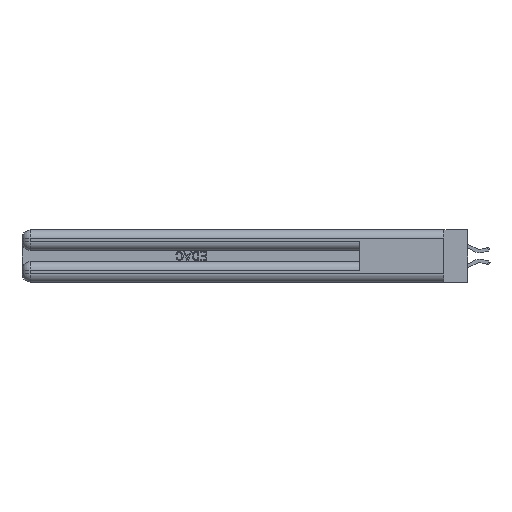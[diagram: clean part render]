
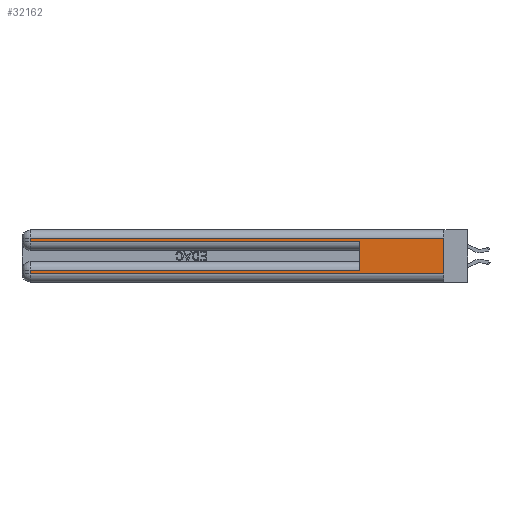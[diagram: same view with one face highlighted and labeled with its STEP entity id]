
A CAD part, left-side view. The second image highlights one B-rep face of the part: STEP entity #32162.
In plain terms, the highlighted planar face has unit normal (-1, 0, 0).
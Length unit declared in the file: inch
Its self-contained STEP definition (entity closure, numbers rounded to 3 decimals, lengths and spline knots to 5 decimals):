
#1844 = DIRECTION ( 'NONE',  ( 0., 0., -1. ) ) ;
#3125 = ORIENTED_EDGE ( 'NONE', *, *, #8062, .T. ) ;
#3623 = ORIENTED_EDGE ( 'NONE', *, *, #20312, .T. ) ;
#4975 = DIRECTION ( 'NONE',  ( 0., 0., -1. ) ) ;
#5886 = AXIS2_PLACEMENT_3D ( 'NONE', #33675, #36899, #17647 ) ;
#6478 = LINE ( 'NONE', #30797, #31210 ) ;
#6628 = LINE ( 'NONE', #17443, #39851 ) ;
#6711 = EDGE_CURVE ( 'NONE', #34396, #38334, #29450, .T. ) ;
#7261 = EDGE_CURVE ( 'NONE', #36686, #39911, #33912, .T. ) ;
#8062 = EDGE_CURVE ( 'NONE', #36686, #34396, #6628, .T. ) ;
#8280 = EDGE_LOOP ( 'NONE', ( #28367, #3623, #14246, #16308, #25900, #3125, #38433, #40405 ) ) ;
#9672 = VECTOR ( 'NONE', #1844, 39.37008 ) ;
#10663 = EDGE_CURVE ( 'NONE', #37939, #33189, #6478, .T. ) ;
#11004 = DIRECTION ( 'NONE',  ( 0., -1., 0. ) ) ;
#11037 = LINE ( 'NONE', #28527, #35695 ) ;
#11185 = PLANE ( 'NONE',  #5886 ) ;
#12347 = DIRECTION ( 'NONE',  ( 0., -1., 0. ) ) ;
#12499 = EDGE_CURVE ( 'NONE', #31010, #18338, #26779, .T. ) ;
#14246 = ORIENTED_EDGE ( 'NONE', *, *, #12499, .T. ) ;
#14874 = VECTOR ( 'NONE', #34053, 39.37008 ) ;
#16308 = ORIENTED_EDGE ( 'NONE', *, *, #22185, .T. ) ;
#17443 = CARTESIAN_POINT ( 'NONE',  ( 0., 0., 0.085 ) ) ;
#17647 = DIRECTION ( 'NONE',  ( 0., 0., -1. ) ) ;
#17827 = CARTESIAN_POINT ( 'NONE',  ( 0., 0.6, 0.145 ) ) ;
#17881 = CARTESIAN_POINT ( 'NONE',  ( 0., 0., 0.31 ) ) ;
#18338 = VERTEX_POINT ( 'NONE', #25374 ) ;
#19590 = CARTESIAN_POINT ( 'NONE',  ( 0., 2.94, 0.31 ) ) ;
#20312 = EDGE_CURVE ( 'NONE', #37939, #31010, #23450, .T. ) ;
#20659 = DIRECTION ( 'NONE',  ( 0., 1., 0. ) ) ;
#20880 = VECTOR ( 'NONE', #40449, 39.37008 ) ;
#22185 = EDGE_CURVE ( 'NONE', #18338, #39911, #30398, .T. ) ;
#22467 = FACE_OUTER_BOUND ( 'NONE', #8280, .T. ) ;
#22581 = CARTESIAN_POINT ( 'NONE',  ( 0., 2.94, 0.085 ) ) ;
#23450 = LINE ( 'NONE', #17881, #14874 ) ;
#23798 = CARTESIAN_POINT ( 'NONE',  ( 0., 0., 0.285 ) ) ;
#24309 = DIRECTION ( 'NONE',  ( 0., 0., 1. ) ) ;
#24623 = CARTESIAN_POINT ( 'NONE',  ( 0., 2.94, 0.37 ) ) ;
#25374 = CARTESIAN_POINT ( 'NONE',  ( 0., 2.94, 0.285 ) ) ;
#25411 = VECTOR ( 'NONE', #24309, 39.37008 ) ;
#25900 = ORIENTED_EDGE ( 'NONE', *, *, #7261, .F. ) ;
#26779 = LINE ( 'NONE', #24623, #9672 ) ;
#28060 = CARTESIAN_POINT ( 'NONE',  ( 0., 0.6, 0.285 ) ) ;
#28367 = ORIENTED_EDGE ( 'NONE', *, *, #10663, .F. ) ;
#28527 = CARTESIAN_POINT ( 'NONE',  ( 0., 0., 0.06 ) ) ;
#29450 = LINE ( 'NONE', #37253, #20880 ) ;
#30398 = LINE ( 'NONE', #23798, #37921 ) ;
#30797 = CARTESIAN_POINT ( 'NONE',  ( 0., 0., 0.37 ) ) ;
#31010 = VERTEX_POINT ( 'NONE', #19590 ) ;
#31210 = VECTOR ( 'NONE', #4975, 39.37008 ) ;
#32162 = ADVANCED_FACE ( 'NONE', ( #22467 ), #11185, .F. ) ;
#33189 = VERTEX_POINT ( 'NONE', #35022 ) ;
#33675 = CARTESIAN_POINT ( 'NONE',  ( 0., 0., 0.37 ) ) ;
#33912 = LINE ( 'NONE', #17827, #25411 ) ;
#34053 = DIRECTION ( 'NONE',  ( 0., 1., 0. ) ) ;
#34396 = VERTEX_POINT ( 'NONE', #22581 ) ;
#34678 = CARTESIAN_POINT ( 'NONE',  ( 0., 0., 0.31 ) ) ;
#35022 = CARTESIAN_POINT ( 'NONE',  ( 0., 0., 0.06 ) ) ;
#35695 = VECTOR ( 'NONE', #12347, 39.37008 ) ;
#36686 = VERTEX_POINT ( 'NONE', #38429 ) ;
#36899 = DIRECTION ( 'NONE',  ( 1., 0., 0. ) ) ;
#37253 = CARTESIAN_POINT ( 'NONE',  ( 0., 2.94, 0.37 ) ) ;
#37921 = VECTOR ( 'NONE', #11004, 39.37008 ) ;
#37939 = VERTEX_POINT ( 'NONE', #34678 ) ;
#38334 = VERTEX_POINT ( 'NONE', #39787 ) ;
#38429 = CARTESIAN_POINT ( 'NONE',  ( 0., 0.6, 0.085 ) ) ;
#38433 = ORIENTED_EDGE ( 'NONE', *, *, #6711, .T. ) ;
#39325 = EDGE_CURVE ( 'NONE', #38334, #33189, #11037, .T. ) ;
#39787 = CARTESIAN_POINT ( 'NONE',  ( 0., 2.94, 0.06 ) ) ;
#39851 = VECTOR ( 'NONE', #20659, 39.37008 ) ;
#39911 = VERTEX_POINT ( 'NONE', #28060 ) ;
#40405 = ORIENTED_EDGE ( 'NONE', *, *, #39325, .T. ) ;
#40449 = DIRECTION ( 'NONE',  ( 0., 0., -1. ) ) ;
